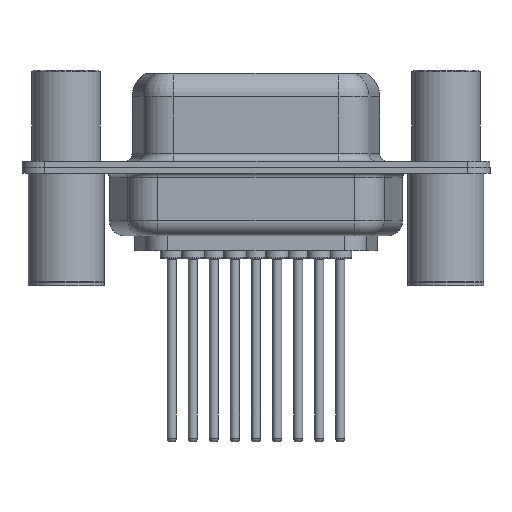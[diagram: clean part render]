
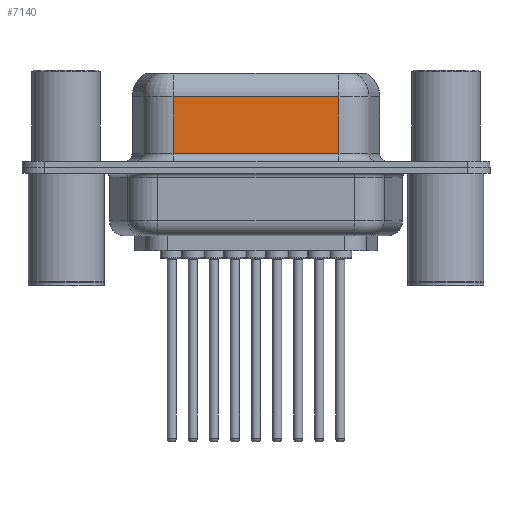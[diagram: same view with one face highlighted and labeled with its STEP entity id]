
A CAD part, front view. The second image highlights one B-rep face of the part: STEP entity #7140.
In plain terms, the highlighted planar face has unit normal (0, -1, 0).
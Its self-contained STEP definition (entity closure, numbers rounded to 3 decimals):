
#879 = DIRECTION ( 'NONE',  ( 0., 0., 1. ) ) ;
#1033 = CARTESIAN_POINT ( 'NONE',  ( 17.962, -3.95, 0.9 ) ) ;
#1240 = EDGE_CURVE ( 'NONE', #15111, #10873, #2756, .T. ) ;
#2409 = VECTOR ( 'NONE', #9514, 1000. ) ;
#2704 = DIRECTION ( 'NONE',  ( 0., 0., -1. ) ) ;
#2756 = LINE ( 'NONE', #6701, #2409 ) ;
#4011 = LINE ( 'NONE', #14763, #4905 ) ;
#4550 = FACE_OUTER_BOUND ( 'NONE', #15710, .T. ) ;
#4905 = VECTOR ( 'NONE', #2704, 1000. ) ;
#5562 = CARTESIAN_POINT ( 'NONE',  ( 17.962, -3.95, 4.65 ) ) ;
#5703 = EDGE_CURVE ( 'NONE', #10905, #10873, #4011, .T. ) ;
#5935 = DIRECTION ( 'NONE',  ( 0., 0., -1. ) ) ;
#6045 = CARTESIAN_POINT ( 'NONE',  ( 17.962, -3.95, 6.4 ) ) ;
#6143 = DIRECTION ( 'NONE',  ( 0., 1., 0. ) ) ;
#6304 = LINE ( 'NONE', #12747, #16741 ) ;
#6638 = VECTOR ( 'NONE', #8279, 1000. ) ;
#6701 = CARTESIAN_POINT ( 'NONE',  ( 17.962, -3.95, 0.9 ) ) ;
#7039 = CARTESIAN_POINT ( 'NONE',  ( 7.038, -3.95, 4.65 ) ) ;
#7127 = LINE ( 'NONE', #5562, #6638 ) ;
#7140 = ADVANCED_FACE ( 'NONE', ( #4550 ), #8856, .F. ) ;
#7374 = ORIENTED_EDGE ( 'NONE', *, *, #16000, .T. ) ;
#8279 = DIRECTION ( 'NONE',  ( -1., 0., 0. ) ) ;
#8755 = EDGE_CURVE ( 'NONE', #10905, #16458, #7127, .T. ) ;
#8856 = PLANE ( 'NONE',  #15041 ) ;
#9514 = DIRECTION ( 'NONE',  ( 1., 0., 0. ) ) ;
#10873 = VERTEX_POINT ( 'NONE', #1033 ) ;
#10905 = VERTEX_POINT ( 'NONE', #10937 ) ;
#10937 = CARTESIAN_POINT ( 'NONE',  ( 17.962, -3.95, 4.65 ) ) ;
#11218 = CARTESIAN_POINT ( 'NONE',  ( 7.038, -3.95, 0.9 ) ) ;
#12747 = CARTESIAN_POINT ( 'NONE',  ( 7.038, -3.95, 6.4 ) ) ;
#12758 = ORIENTED_EDGE ( 'NONE', *, *, #5703, .F. ) ;
#14763 = CARTESIAN_POINT ( 'NONE',  ( 17.962, -3.95, 6.4 ) ) ;
#15041 = AXIS2_PLACEMENT_3D ( 'NONE', #6045, #6143, #879 ) ;
#15111 = VERTEX_POINT ( 'NONE', #11218 ) ;
#15213 = ORIENTED_EDGE ( 'NONE', *, *, #8755, .T. ) ;
#15710 = EDGE_LOOP ( 'NONE', ( #12758, #15213, #7374, #16079 ) ) ;
#16000 = EDGE_CURVE ( 'NONE', #16458, #15111, #6304, .T. ) ;
#16079 = ORIENTED_EDGE ( 'NONE', *, *, #1240, .T. ) ;
#16458 = VERTEX_POINT ( 'NONE', #7039 ) ;
#16741 = VECTOR ( 'NONE', #5935, 1000. ) ;
